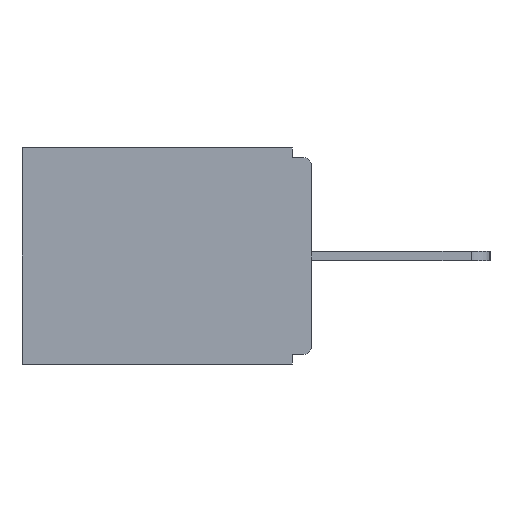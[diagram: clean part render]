
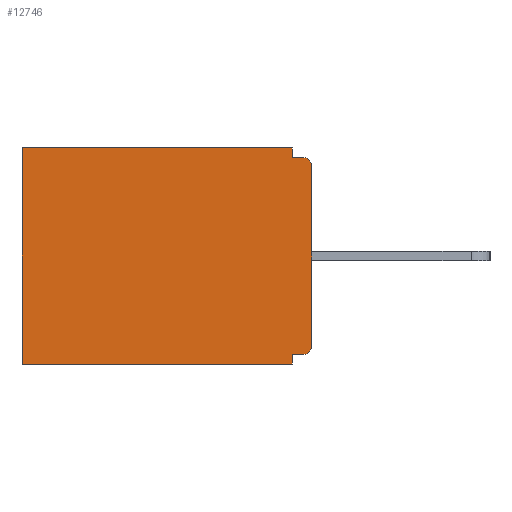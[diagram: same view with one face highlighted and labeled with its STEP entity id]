
A CAD part, left-side view. The second image highlights one B-rep face of the part: STEP entity #12746.
In plain terms, the highlighted planar face has unit normal (-1, 0, 0).
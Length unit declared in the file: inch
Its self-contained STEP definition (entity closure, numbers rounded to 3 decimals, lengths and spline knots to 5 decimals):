
#141 = DIRECTION ( 'NONE',  ( 0., -1., 0. ) ) ;
#279 = FACE_OUTER_BOUND ( 'NONE', #10554, .T. ) ;
#381 = CARTESIAN_POINT ( 'NONE',  ( 0.298, 0., -0.328 ) ) ;
#543 = CARTESIAN_POINT ( 'NONE',  ( 0.298, 0.031, -0.343 ) ) ;
#589 = EDGE_CURVE ( 'NONE', #1489, #8592, #7019, .T. ) ;
#913 = DIRECTION ( 'NONE',  ( -1., 0., 0. ) ) ;
#1037 = ORIENTED_EDGE ( 'NONE', *, *, #9787, .F. ) ;
#1430 = VECTOR ( 'NONE', #12953, 39.37008 ) ;
#1489 = VERTEX_POINT ( 'NONE', #10068 ) ;
#1543 = EDGE_CURVE ( 'NONE', #13304, #6231, #2016, .T. ) ;
#1869 = CARTESIAN_POINT ( 'NONE',  ( 0.298, 0.031, 0. ) ) ;
#2012 = ORIENTED_EDGE ( 'NONE', *, *, #589, .F. ) ;
#2016 = LINE ( 'NONE', #12720, #10561 ) ;
#2651 = ORIENTED_EDGE ( 'NONE', *, *, #6500, .T. ) ;
#2778 = VECTOR ( 'NONE', #9545, 39.37008 ) ;
#3028 = DIRECTION ( 'NONE',  ( 0., 0., -1. ) ) ;
#3249 = DIRECTION ( 'NONE',  ( 0., 0., -1. ) ) ;
#3545 = CARTESIAN_POINT ( 'NONE',  ( 0.298, 0.015, -0.313 ) ) ;
#3765 = CIRCLE ( 'NONE', #7069, 0.015 ) ;
#3887 = VECTOR ( 'NONE', #9014, 39.37008 ) ;
#4152 = EDGE_CURVE ( 'NONE', #8091, #7798, #3765, .T. ) ;
#4492 = ORIENTED_EDGE ( 'NONE', *, *, #5094, .F. ) ;
#4679 = LINE ( 'NONE', #543, #10465 ) ;
#4789 = VERTEX_POINT ( 'NONE', #1869 ) ;
#5034 = CARTESIAN_POINT ( 'NONE',  ( 0.298, 0.031, -0.328 ) ) ;
#5094 = EDGE_CURVE ( 'NONE', #8592, #13304, #4679, .T. ) ;
#5200 = CARTESIAN_POINT ( 'NONE',  ( 0.298, 0., -0.313 ) ) ;
#5225 = LINE ( 'NONE', #14029, #9953 ) ;
#5447 = CARTESIAN_POINT ( 'NONE',  ( 0.298, 0.031, -0.343 ) ) ;
#5572 = AXIS2_PLACEMENT_3D ( 'NONE', #13766, #7021, #14839 ) ;
#5823 = PLANE ( 'NONE',  #5572 ) ;
#5869 = DIRECTION ( 'NONE',  ( 0., 0., -1. ) ) ;
#6018 = CARTESIAN_POINT ( 'NONE',  ( 0.298, 0., 0. ) ) ;
#6231 = VERTEX_POINT ( 'NONE', #7218 ) ;
#6500 = EDGE_CURVE ( 'NONE', #1489, #13045, #10424, .T. ) ;
#6617 = EDGE_CURVE ( 'NONE', #7580, #6231, #14885, .T. ) ;
#6774 = ORIENTED_EDGE ( 'NONE', *, *, #8569, .F. ) ;
#7019 = LINE ( 'NONE', #381, #3887 ) ;
#7021 = DIRECTION ( 'NONE',  ( 1., 0., 0. ) ) ;
#7069 = AXIS2_PLACEMENT_3D ( 'NONE', #13056, #913, #3249 ) ;
#7094 = CARTESIAN_POINT ( 'NONE',  ( 0.298, 0.46, 0. ) ) ;
#7218 = CARTESIAN_POINT ( 'NONE',  ( 0.298, 0.46, -0.343 ) ) ;
#7225 = DIRECTION ( 'NONE',  ( 0., 1., 0. ) ) ;
#7233 = ORIENTED_EDGE ( 'NONE', *, *, #14941, .T. ) ;
#7580 = VERTEX_POINT ( 'NONE', #13333 ) ;
#7798 = VERTEX_POINT ( 'NONE', #14752 ) ;
#8091 = VERTEX_POINT ( 'NONE', #8650 ) ;
#8421 = VECTOR ( 'NONE', #7225, 39.37008 ) ;
#8569 = EDGE_CURVE ( 'NONE', #8091, #13045, #10722, .T. ) ;
#8592 = VERTEX_POINT ( 'NONE', #5034 ) ;
#8650 = CARTESIAN_POINT ( 'NONE',  ( 0.298, 0., -0.03 ) ) ;
#8799 = DIRECTION ( 'NONE',  ( 0., 1., 0. ) ) ;
#9014 = DIRECTION ( 'NONE',  ( 0., 1., 0. ) ) ;
#9040 = CARTESIAN_POINT ( 'NONE',  ( 0.298, 0.031, -0.015 ) ) ;
#9049 = ORIENTED_EDGE ( 'NONE', *, *, #1543, .F. ) ;
#9488 = VECTOR ( 'NONE', #5869, 39.37008 ) ;
#9545 = DIRECTION ( 'NONE',  ( 0., 0., -1. ) ) ;
#9687 = ORIENTED_EDGE ( 'NONE', *, *, #6617, .T. ) ;
#9787 = EDGE_CURVE ( 'NONE', #4789, #13956, #12076, .T. ) ;
#9953 = VECTOR ( 'NONE', #141, 39.37008 ) ;
#10068 = CARTESIAN_POINT ( 'NONE',  ( 0.298, 0.015, -0.328 ) ) ;
#10424 = CIRCLE ( 'NONE', #11648, 0.015 ) ;
#10465 = VECTOR ( 'NONE', #3028, 39.37008 ) ;
#10554 = EDGE_LOOP ( 'NONE', ( #10808, #13475, #1037, #7233, #9687, #9049, #4492, #2012, #2651, #6774 ) ) ;
#10561 = VECTOR ( 'NONE', #8799, 39.37008 ) ;
#10722 = LINE ( 'NONE', #11848, #1430 ) ;
#10808 = ORIENTED_EDGE ( 'NONE', *, *, #4152, .T. ) ;
#11056 = DIRECTION ( 'NONE',  ( 0., 0., -1. ) ) ;
#11084 = EDGE_CURVE ( 'NONE', #13956, #7798, #5225, .T. ) ;
#11648 = AXIS2_PLACEMENT_3D ( 'NONE', #3545, #14725, #11056 ) ;
#11848 = CARTESIAN_POINT ( 'NONE',  ( 0.298, 0., 0. ) ) ;
#12076 = LINE ( 'NONE', #12698, #9488 ) ;
#12698 = CARTESIAN_POINT ( 'NONE',  ( 0.298, 0.031, -0.343 ) ) ;
#12720 = CARTESIAN_POINT ( 'NONE',  ( 0.298, 0., -0.343 ) ) ;
#12746 = ADVANCED_FACE ( 'NONE', ( #279 ), #5823, .F. ) ;
#12953 = DIRECTION ( 'NONE',  ( 0., 0., -1. ) ) ;
#13045 = VERTEX_POINT ( 'NONE', #5200 ) ;
#13056 = CARTESIAN_POINT ( 'NONE',  ( 0.298, 0.015, -0.03 ) ) ;
#13304 = VERTEX_POINT ( 'NONE', #5447 ) ;
#13333 = CARTESIAN_POINT ( 'NONE',  ( 0.298, 0.46, 0. ) ) ;
#13475 = ORIENTED_EDGE ( 'NONE', *, *, #11084, .F. ) ;
#13766 = CARTESIAN_POINT ( 'NONE',  ( 0.298, 0., 0. ) ) ;
#13956 = VERTEX_POINT ( 'NONE', #9040 ) ;
#14029 = CARTESIAN_POINT ( 'NONE',  ( 0.298, 0., -0.015 ) ) ;
#14328 = LINE ( 'NONE', #6018, #8421 ) ;
#14725 = DIRECTION ( 'NONE',  ( -1., 0., 0. ) ) ;
#14752 = CARTESIAN_POINT ( 'NONE',  ( 0.298, 0.015, -0.015 ) ) ;
#14839 = DIRECTION ( 'NONE',  ( 0., 0., -1. ) ) ;
#14885 = LINE ( 'NONE', #7094, #2778 ) ;
#14941 = EDGE_CURVE ( 'NONE', #4789, #7580, #14328, .T. ) ;
